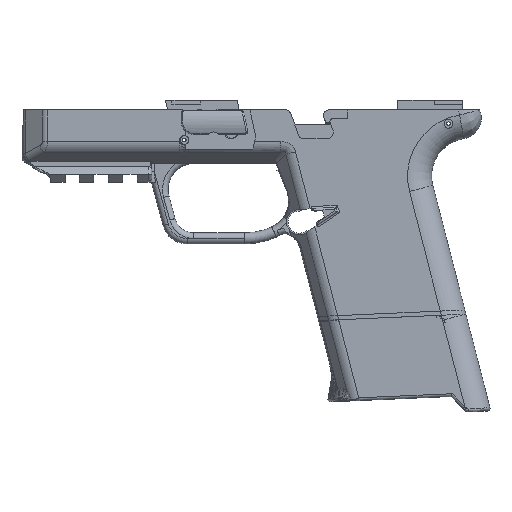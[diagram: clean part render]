
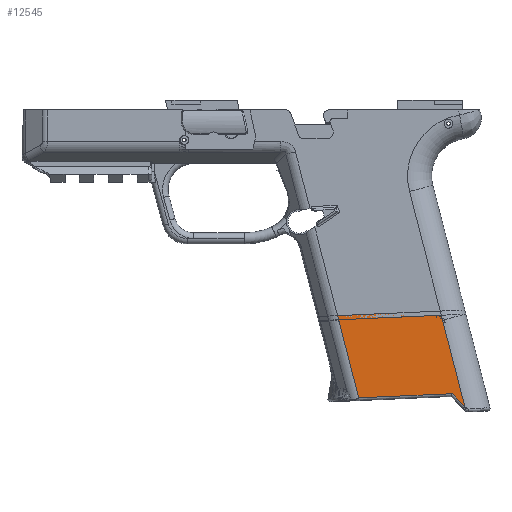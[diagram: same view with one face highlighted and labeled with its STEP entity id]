
A CAD part, left-side view. The second image highlights one B-rep face of the part: STEP entity #12545.
In plain terms, the highlighted face is planar.
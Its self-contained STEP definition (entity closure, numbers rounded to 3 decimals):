
#1043=PLANE('',#13750);
#1717=FACE_OUTER_BOUND('',#2443,.T.);
#2443=EDGE_LOOP('',(#11549,#11550,#11551,#11552,#11553));
#3478=LINE('',#24312,#4557);
#3498=LINE('',#25158,#4577);
#3512=LINE('',#25579,#4591);
#3513=LINE('',#25583,#4592);
#3514=LINE('',#25584,#4593);
#4557=VECTOR('',#16827,10.);
#4577=VECTOR('',#16919,10.);
#4591=VECTOR('',#16991,10.);
#4592=VECTOR('',#16996,10.);
#4593=VECTOR('',#16997,10.);
#6035=VERTEX_POINT('',#24290);
#6037=VERTEX_POINT('',#24310);
#6091=VERTEX_POINT('',#25157);
#6110=VERTEX_POINT('',#25420);
#6118=VERTEX_POINT('',#25582);
#7814=EDGE_CURVE('',#6037,#6035,#3478,.T.);
#7896=EDGE_CURVE('',#6091,#6035,#3498,.T.);
#7941=EDGE_CURVE('',#6110,#6037,#3512,.T.);
#7942=EDGE_CURVE('',#6118,#6110,#3513,.T.);
#7943=EDGE_CURVE('',#6118,#6091,#3514,.T.);
#11549=ORIENTED_EDGE('',*,*,#7814,.F.);
#11550=ORIENTED_EDGE('',*,*,#7941,.F.);
#11551=ORIENTED_EDGE('',*,*,#7942,.F.);
#11552=ORIENTED_EDGE('',*,*,#7943,.T.);
#11553=ORIENTED_EDGE('',*,*,#7896,.T.);
#12545=ADVANCED_FACE('',(#1717),#1043,.T.);
#13750=AXIS2_PLACEMENT_3D('',#25581,#16994,#16995);
#16827=DIRECTION('',(0.,0.999,0.044));
#16919=DIRECTION('',(0.,-0.249,0.969));
#16991=DIRECTION('',(0.,0.697,-0.717));
#16994=DIRECTION('center_axis',(1.,0.,0.));
#16995=DIRECTION('ref_axis',(0.,0.999,0.044));
#16996=DIRECTION('',(0.,-0.249,0.969));
#16997=DIRECTION('',(0.,0.999,0.044));
#24290=CARTESIAN_POINT('',(22.175,-44.727,96.906));
#24310=CARTESIAN_POINT('',(22.175,-78.67,95.402));
#24312=CARTESIAN_POINT('',(22.175,-44.598,96.911));
#25157=CARTESIAN_POINT('',(22.175,-37.062,67.087));
#25158=CARTESIAN_POINT('',(22.175,-37.062,67.087));
#25420=CARTESIAN_POINT('',(22.175,-83.249,100.107));
#25579=CARTESIAN_POINT('',(22.175,-73.025,89.603));
#25581=CARTESIAN_POINT('Origin',(22.175,-74.337,65.435));
#25582=CARTESIAN_POINT('',(22.175,-74.337,65.435));
#25583=CARTESIAN_POINT('',(22.175,-74.337,65.435));
#25584=CARTESIAN_POINT('',(22.175,-40.4,66.939));
